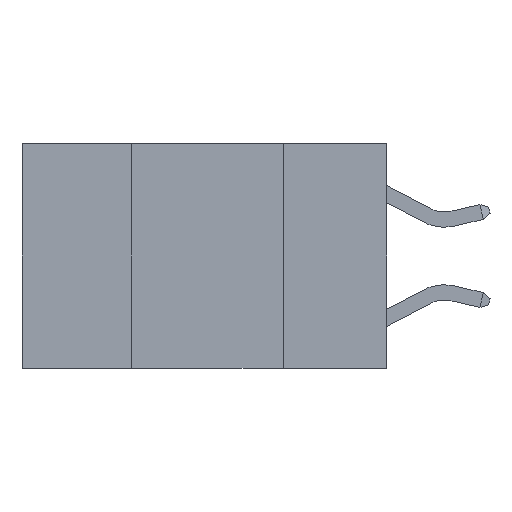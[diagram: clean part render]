
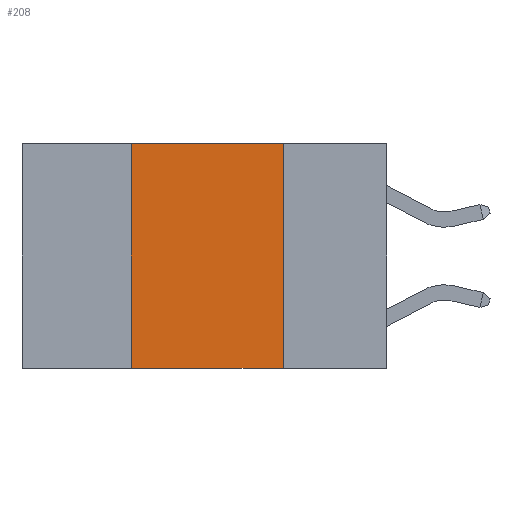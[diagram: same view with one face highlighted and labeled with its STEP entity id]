
A CAD part, left-side view. The second image highlights one B-rep face of the part: STEP entity #208.
In plain terms, the highlighted planar face has unit normal (-1, 0, 0).
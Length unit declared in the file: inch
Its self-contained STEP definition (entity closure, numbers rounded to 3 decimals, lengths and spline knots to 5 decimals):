
#208 = ADVANCED_FACE ( 'NONE', ( #23445 ), #14696, .F. ) ;
#1612 = CARTESIAN_POINT ( 'NONE',  ( 0., 0.6, 0. ) ) ;
#3300 = DIRECTION ( 'NONE',  ( 1., 0., 0. ) ) ;
#3587 = CARTESIAN_POINT ( 'NONE',  ( 0., 0.42, -0.37 ) ) ;
#4435 = CARTESIAN_POINT ( 'NONE',  ( 0., 0.17, 0. ) ) ;
#5010 = LINE ( 'NONE', #4435, #16300 ) ;
#8051 = CARTESIAN_POINT ( 'NONE',  ( 0., 0.42, 0. ) ) ;
#9075 = CARTESIAN_POINT ( 'NONE',  ( 0., 0.6, -0.37 ) ) ;
#10473 = CARTESIAN_POINT ( 'NONE',  ( 0., 0.17, 0. ) ) ;
#11238 = VECTOR ( 'NONE', #24131, 39.37008 ) ;
#11303 = LINE ( 'NONE', #9075, #22453 ) ;
#11899 = VERTEX_POINT ( 'NONE', #8051 ) ;
#12300 = VERTEX_POINT ( 'NONE', #23452 ) ;
#13212 = CARTESIAN_POINT ( 'NONE',  ( 0., 0.42, 0. ) ) ;
#14517 = AXIS2_PLACEMENT_3D ( 'NONE', #14845, #3300, #25974 ) ;
#14696 = PLANE ( 'NONE',  #14517 ) ;
#14845 = CARTESIAN_POINT ( 'NONE',  ( 0., 0.6, 0. ) ) ;
#15464 = DIRECTION ( 'NONE',  ( 0., -1., 0. ) ) ;
#15473 = VERTEX_POINT ( 'NONE', #3587 ) ;
#16300 = VECTOR ( 'NONE', #29162, 39.37008 ) ;
#16828 = ORIENTED_EDGE ( 'NONE', *, *, #19110, .F. ) ;
#18624 = EDGE_CURVE ( 'NONE', #15473, #12300, #11303, .T. ) ;
#19110 = EDGE_CURVE ( 'NONE', #26216, #12300, #5010, .T. ) ;
#20295 = EDGE_CURVE ( 'NONE', #15473, #11899, #22257, .T. ) ;
#21894 = EDGE_CURVE ( 'NONE', #11899, #26216, #21925, .T. ) ;
#21925 = LINE ( 'NONE', #1612, #11238 ) ;
#22257 = LINE ( 'NONE', #13212, #23465 ) ;
#22453 = VECTOR ( 'NONE', #15464, 39.37008 ) ;
#22724 = ORIENTED_EDGE ( 'NONE', *, *, #20295, .F. ) ;
#23445 = FACE_OUTER_BOUND ( 'NONE', #27020, .T. ) ;
#23452 = CARTESIAN_POINT ( 'NONE',  ( 0., 0.17, -0.37 ) ) ;
#23465 = VECTOR ( 'NONE', #26698, 39.37008 ) ;
#24131 = DIRECTION ( 'NONE',  ( 0., -1., 0. ) ) ;
#25974 = DIRECTION ( 'NONE',  ( 0., 0., -1. ) ) ;
#26216 = VERTEX_POINT ( 'NONE', #10473 ) ;
#26698 = DIRECTION ( 'NONE',  ( 0., 0., 1. ) ) ;
#26725 = ORIENTED_EDGE ( 'NONE', *, *, #21894, .F. ) ;
#27020 = EDGE_LOOP ( 'NONE', ( #16828, #26725, #22724, #28362 ) ) ;
#28362 = ORIENTED_EDGE ( 'NONE', *, *, #18624, .T. ) ;
#29162 = DIRECTION ( 'NONE',  ( 0., 0., -1. ) ) ;
